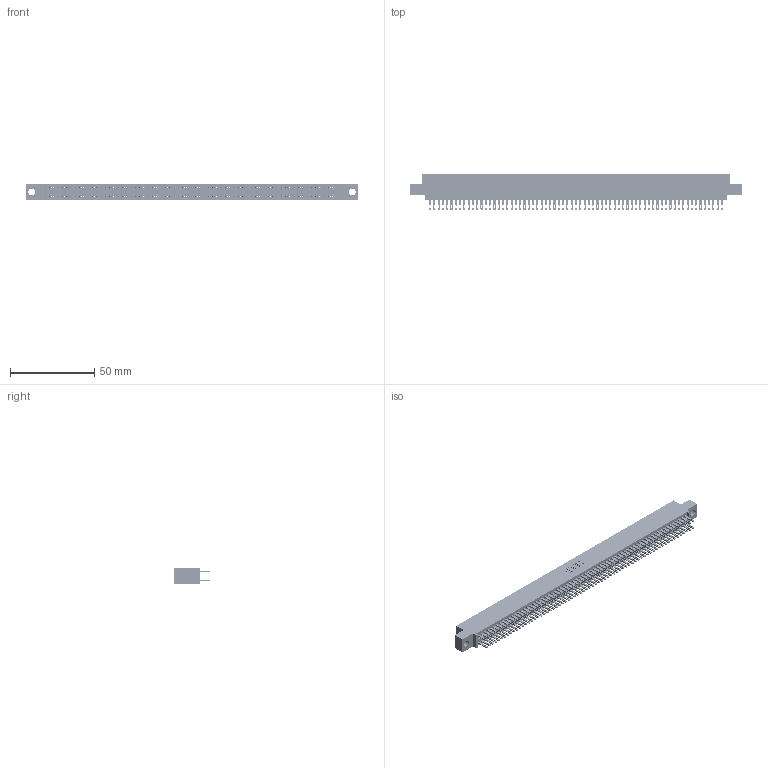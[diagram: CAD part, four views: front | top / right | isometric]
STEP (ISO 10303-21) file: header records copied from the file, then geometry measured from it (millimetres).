
FILE_DESCRIPTION (( 'STEP AP203' ), '1' );
FILE_NAME ('895-138-500-504.STEP', '2020-10-13T18:57:41', ( '' ), ( '' ), 'SwSTEP 2.0', 'SolidWorks 2020', '' );
FILE_SCHEMA (( 'CONFIG_CONTROL_DESIGN' ));
Length unit declared in the file: inch
Products named in the file (3): 895-138-500-504; 845 Part_0.110 Offset - 0.156 Dia-TH; 345-292-001_345-293-100
Assembly tree (139 placements, depth 2):
  895-138-500-504
    845 Part_0.110 Offset - 0.156 Dia-TH
    345-292-001_345-293-100  x138
Bounding box: 196.47 x 21.51 x 9.4 mm (x, y, z)
Volume: 19596.3 mm3; surface area: 30805.1 mm2
Topology: 139 solids, 139 shells, 6478 faces, 19811 edges, 13206 vertices
Faces by surface type: plane 3810, cylinder 2668
Entity records: 50569 total; most frequent: CARTESIAN_POINT 8452, ORIENTED_EDGE 8386, DIRECTION 7421, EDGE_CURVE 4193, VECTOR 3781, LINE 3781, VERTEX_POINT 2794, AXIS2_PLACEMENT_3D 1820
